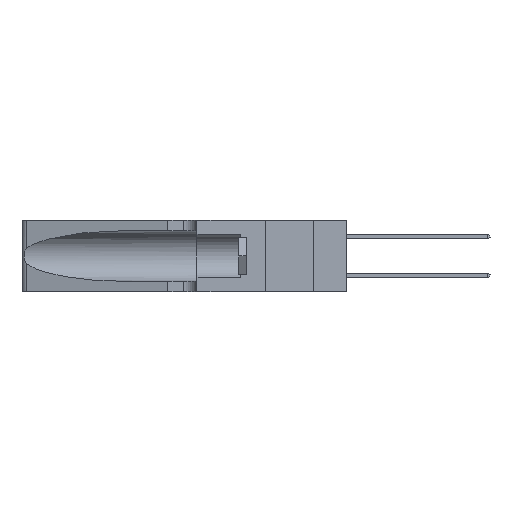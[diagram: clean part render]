
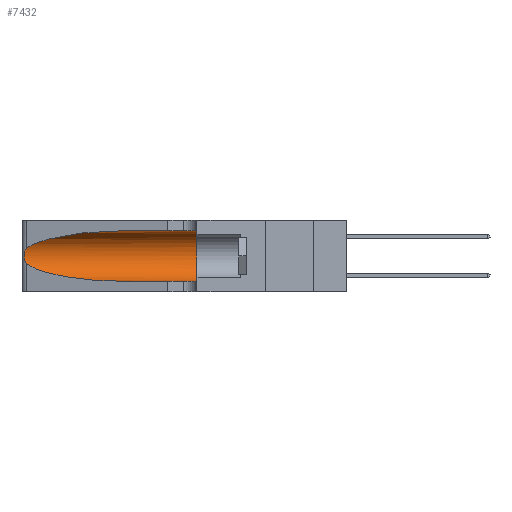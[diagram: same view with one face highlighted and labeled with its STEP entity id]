
A CAD part, left-side view. The second image highlights one B-rep face of the part: STEP entity #7432.
In plain terms, the highlighted cylindrical face has radius 3.308 mm (diameter 6.617 mm), a partial arc.
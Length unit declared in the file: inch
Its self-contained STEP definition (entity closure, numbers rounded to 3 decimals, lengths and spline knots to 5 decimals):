
#208 = VERTEX_POINT ( 'NONE', #5810 ) ;
#416 = CARTESIAN_POINT ( 'NONE',  ( 0.2373, 1.15595, 0.28018 ) ) ;
#1722 = DIRECTION ( 'NONE',  ( 0., 1., 0. ) ) ;
#1879 = VERTEX_POINT ( 'NONE', #28670 ) ;
#2056 = CARTESIAN_POINT ( 'NONE',  ( 0.25487, 1.22718, 0.14631 ) ) ;
#2774 = CARTESIAN_POINT ( 'NONE',  ( 0.25789, 1.23486, 0.15765 ) ) ;
#4369 = B_SPLINE_CURVE_WITH_KNOTS ( 'NONE', 3,
 ( #23873, #26900, #29906, #11844, #32919, #14883, #35958, #17905, #38961, #20965, #2774, #23997, #5900, #27036 ),
 .UNSPECIFIED., .F., .F.,
 ( 4, 2, 2, 2, 2, 2, 4 ),
 ( 0., 0.00027, 0.00053, 0.00107, 0.0016, 0.00187, 0.00214 ),
 .UNSPECIFIED. ) ;
#5620 = EDGE_LOOP ( 'NONE', ( #37306, #28412, #15869, #6367, #26134, #8431 ) ) ;
#5810 = CARTESIAN_POINT ( 'NONE',  ( 0.1305, 0.35, 0.31525 ) ) ;
#5900 = CARTESIAN_POINT ( 'NONE',  ( 0.25555, 1.22993, 0.14849 ) ) ;
#6204 =( BOUNDED_CURVE ( )  B_SPLINE_CURVE ( 3, ( #9540, #30621, #416, #21718 ),
 .UNSPECIFIED., .F., .F. ) 
 B_SPLINE_CURVE_WITH_KNOTS ( ( 4, 4 ),
 ( 1.5708, 2.84003 ),
 .UNSPECIFIED. ) 
 CURVE ( )  GEOMETRIC_REPRESENTATION_ITEM ( )  RATIONAL_B_SPLINE_CURVE ( ( 1., 0.87, 0.87, 1. ) ) 
 REPRESENTATION_ITEM ( '' )  );
#6367 = ORIENTED_EDGE ( 'NONE', *, *, #23880, .T. ) ;
#6598 = CARTESIAN_POINT ( 'NONE',  ( 0.1305, 0.72297, 0.31525 ) ) ;
#7432 = ADVANCED_FACE ( 'NONE', ( #35378 ), #11351, .F. ) ;
#8108 = CIRCLE ( 'NONE', #17104, 0.13025 ) ;
#8262 = CARTESIAN_POINT ( 'NONE',  ( 0.1305, 0.72297, 0.05475 ) ) ;
#8431 = ORIENTED_EDGE ( 'NONE', *, *, #10262, .F. ) ;
#9540 = CARTESIAN_POINT ( 'NONE',  ( 0.1305, 0.72297, 0.31525 ) ) ;
#10262 = EDGE_CURVE ( 'NONE', #20216, #208, #23945, .T. ) ;
#10590 = AXIS2_PLACEMENT_3D ( 'NONE', #20392, #29218, #17334 ) ;
#11351 = CYLINDRICAL_SURFACE ( 'NONE', #10590, 0.13025 ) ;
#11389 = DIRECTION ( 'NONE',  ( 0., -1., 0. ) ) ;
#11844 = CARTESIAN_POINT ( 'NONE',  ( 0.25787, 1.23484, 0.2124 ) ) ;
#14259 = CARTESIAN_POINT ( 'NONE',  ( 0.1305, 0.72297, 0.05475 ) ) ;
#14883 = CARTESIAN_POINT ( 'NONE',  ( 0.26018, 1.23835, 0.19895 ) ) ;
#15136 = LINE ( 'NONE', #26426, #23184 ) ;
#15869 = ORIENTED_EDGE ( 'NONE', *, *, #38420, .T. ) ;
#15874 = VECTOR ( 'NONE', #37209, 39.37008 ) ;
#17104 = AXIS2_PLACEMENT_3D ( 'NONE', #19952, #1722, #22991 ) ;
#17334 = DIRECTION ( 'NONE',  ( 0., 0., -1. ) ) ;
#17905 = CARTESIAN_POINT ( 'NONE',  ( 0.26075, 1.23896, 0.178 ) ) ;
#19952 = CARTESIAN_POINT ( 'NONE',  ( 0.1305, 0.35, 0.185 ) ) ;
#20216 = VERTEX_POINT ( 'NONE', #6598 ) ;
#20392 = CARTESIAN_POINT ( 'NONE',  ( 0.1305, 1.61858, 0.185 ) ) ;
#20965 = CARTESIAN_POINT ( 'NONE',  ( 0.25856, 1.23593, 0.16098 ) ) ;
#21491 = CARTESIAN_POINT ( 'NONE',  ( 0.25487, 1.22718, 0.22369 ) ) ;
#21667 = EDGE_CURVE ( 'NONE', #20216, #29563, #6204, .T. ) ;
#21718 = CARTESIAN_POINT ( 'NONE',  ( 0.25487, 1.22718, 0.22369 ) ) ;
#22132 = CARTESIAN_POINT ( 'NONE',  ( 0.1305, 1.61858, 0.31525 ) ) ;
#22991 = DIRECTION ( 'NONE',  ( 0., 0., 1. ) ) ;
#23184 = VECTOR ( 'NONE', #11389, 39.37008 ) ;
#23294 = CARTESIAN_POINT ( 'NONE',  ( 0.2373, 1.15595, 0.08982 ) ) ;
#23873 = CARTESIAN_POINT ( 'NONE',  ( 0.25487, 1.22718, 0.22369 ) ) ;
#23880 = EDGE_CURVE ( 'NONE', #30712, #1879, #15136, .T. ) ;
#23945 = LINE ( 'NONE', #22132, #15874 ) ;
#23997 = CARTESIAN_POINT ( 'NONE',  ( 0.25639, 1.23186, 0.15144 ) ) ;
#24194 = VERTEX_POINT ( 'NONE', #27724 ) ;
#24322 =( BOUNDED_CURVE ( )  B_SPLINE_CURVE ( 3, ( #2056, #23294, #26330, #8262 ),
 .UNSPECIFIED., .F., .F. ) 
 B_SPLINE_CURVE_WITH_KNOTS ( ( 4, 4 ),
 ( 3.44316, 4.71239 ),
 .UNSPECIFIED. ) 
 CURVE ( )  GEOMETRIC_REPRESENTATION_ITEM ( )  RATIONAL_B_SPLINE_CURVE ( ( 1., 0.87, 0.87, 1. ) ) 
 REPRESENTATION_ITEM ( '' )  );
#26134 = ORIENTED_EDGE ( 'NONE', *, *, #34259, .F. ) ;
#26330 = CARTESIAN_POINT ( 'NONE',  ( 0.18966, 0.96281, 0.05475 ) ) ;
#26426 = CARTESIAN_POINT ( 'NONE',  ( 0.1305, 1.61858, 0.05475 ) ) ;
#26900 = CARTESIAN_POINT ( 'NONE',  ( 0.25555, 1.22994, 0.2215 ) ) ;
#27036 = CARTESIAN_POINT ( 'NONE',  ( 0.25487, 1.22718, 0.14631 ) ) ;
#27724 = CARTESIAN_POINT ( 'NONE',  ( 0.25487, 1.22718, 0.14631 ) ) ;
#28412 = ORIENTED_EDGE ( 'NONE', *, *, #37909, .T. ) ;
#28670 = CARTESIAN_POINT ( 'NONE',  ( 0.1305, 0.35, 0.05475 ) ) ;
#29218 = DIRECTION ( 'NONE',  ( 0., -1., 0. ) ) ;
#29563 = VERTEX_POINT ( 'NONE', #21491 ) ;
#29906 = CARTESIAN_POINT ( 'NONE',  ( 0.25639, 1.23184, 0.21858 ) ) ;
#30621 = CARTESIAN_POINT ( 'NONE',  ( 0.18966, 0.96281, 0.31525 ) ) ;
#30712 = VERTEX_POINT ( 'NONE', #14259 ) ;
#32919 = CARTESIAN_POINT ( 'NONE',  ( 0.25854, 1.2359, 0.20912 ) ) ;
#34259 = EDGE_CURVE ( 'NONE', #208, #1879, #8108, .T. ) ;
#35378 = FACE_OUTER_BOUND ( 'NONE', #5620, .T. ) ;
#35958 = CARTESIAN_POINT ( 'NONE',  ( 0.26075, 1.23896, 0.19203 ) ) ;
#37209 = DIRECTION ( 'NONE',  ( 0., -1., 0. ) ) ;
#37306 = ORIENTED_EDGE ( 'NONE', *, *, #21667, .T. ) ;
#37909 = EDGE_CURVE ( 'NONE', #29563, #24194, #4369, .T. ) ;
#38420 = EDGE_CURVE ( 'NONE', #24194, #30712, #24322, .T. ) ;
#38961 = CARTESIAN_POINT ( 'NONE',  ( 0.26017, 1.23833, 0.17102 ) ) ;
